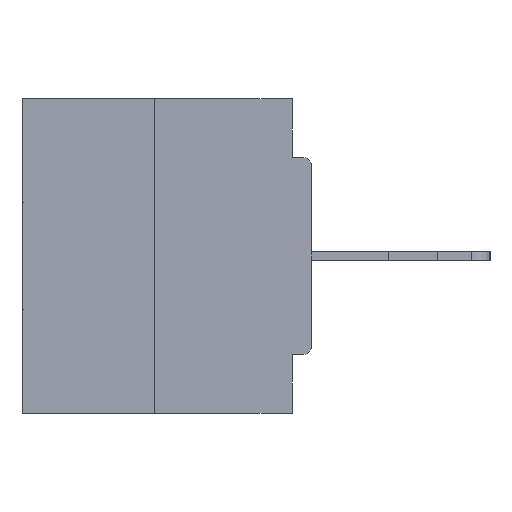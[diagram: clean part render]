
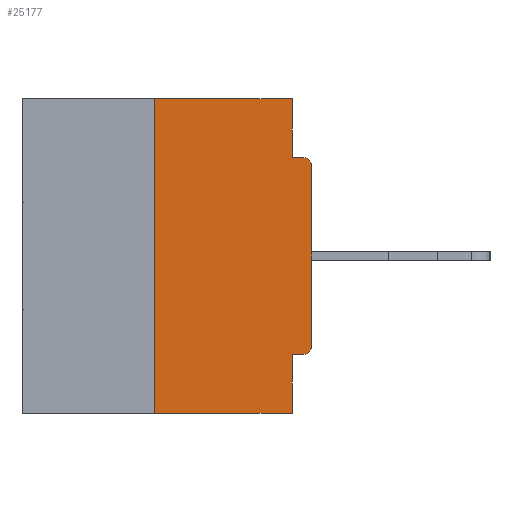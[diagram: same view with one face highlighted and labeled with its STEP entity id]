
A CAD part, left-side view. The second image highlights one B-rep face of the part: STEP entity #25177.
In plain terms, the highlighted planar face has unit normal (-1, 0, 0).
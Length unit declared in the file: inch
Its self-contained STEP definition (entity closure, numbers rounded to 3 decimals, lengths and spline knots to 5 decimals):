
#40 = EDGE_CURVE ( 'NONE', #13439, #9041, #28304, .T. ) ;
#53 = CARTESIAN_POINT ( 'NONE',  ( 0., 0.031, 0. ) ) ;
#135 = ORIENTED_EDGE ( 'NONE', *, *, #31117, .F. ) ;
#334 = CARTESIAN_POINT ( 'NONE',  ( 0., 0.031, 0. ) ) ;
#737 = EDGE_CURVE ( 'NONE', #1061, #24959, #9165, .T. ) ;
#854 = EDGE_CURVE ( 'NONE', #18904, #9041, #8655, .T. ) ;
#1061 = VERTEX_POINT ( 'NONE', #24349 ) ;
#1246 = DIRECTION ( 'NONE',  ( 0., 0., -1. ) ) ;
#1513 = VECTOR ( 'NONE', #6219, 39.37008 ) ;
#1588 = VECTOR ( 'NONE', #11652, 39.37008 ) ;
#2997 = EDGE_LOOP ( 'NONE', ( #18141, #19360, #4685, #22809, #18071, #13295, #12300, #4319, #24448, #135 ) ) ;
#3257 = DIRECTION ( 'NONE',  ( 0., 0., 1. ) ) ;
#4319 = ORIENTED_EDGE ( 'NONE', *, *, #25153, .T. ) ;
#4685 = ORIENTED_EDGE ( 'NONE', *, *, #854, .T. ) ;
#5318 = DIRECTION ( 'NONE',  ( 0., 0., -1. ) ) ;
#5528 = LINE ( 'NONE', #16501, #17212 ) ;
#6044 = CARTESIAN_POINT ( 'NONE',  ( 0., 0.46, -0.5 ) ) ;
#6219 = DIRECTION ( 'NONE',  ( 0., -1., 0. ) ) ;
#7610 = CARTESIAN_POINT ( 'NONE',  ( 0., 0., -0.4065 ) ) ;
#8655 = LINE ( 'NONE', #6044, #16555 ) ;
#9040 = VECTOR ( 'NONE', #1246, 39.37008 ) ;
#9041 = VERTEX_POINT ( 'NONE', #32996 ) ;
#9165 = LINE ( 'NONE', #25255, #1513 ) ;
#9219 = CARTESIAN_POINT ( 'NONE',  ( 0., 0., 0. ) ) ;
#9631 = CARTESIAN_POINT ( 'NONE',  ( 0., 0.25, -0.5 ) ) ;
#9983 = EDGE_CURVE ( 'NONE', #22414, #21853, #27924, .T. ) ;
#10182 = VECTOR ( 'NONE', #23954, 39.37008 ) ;
#10541 = CARTESIAN_POINT ( 'NONE',  ( 0., 0.015, -0.3915 ) ) ;
#11055 = VERTEX_POINT ( 'NONE', #11206 ) ;
#11206 = CARTESIAN_POINT ( 'NONE',  ( 0., 0.25, 0. ) ) ;
#11652 = DIRECTION ( 'NONE',  ( 0., 0., -1. ) ) ;
#11832 = DIRECTION ( 'NONE',  ( 0., 0., 1. ) ) ;
#12300 = ORIENTED_EDGE ( 'NONE', *, *, #9983, .T. ) ;
#13295 = ORIENTED_EDGE ( 'NONE', *, *, #13466, .T. ) ;
#13439 = VERTEX_POINT ( 'NONE', #15628 ) ;
#13466 = EDGE_CURVE ( 'NONE', #27316, #22414, #32610, .T. ) ;
#13702 = DIRECTION ( 'NONE',  ( 0., 1., 0. ) ) ;
#14449 = LINE ( 'NONE', #53, #1588 ) ;
#15037 = CARTESIAN_POINT ( 'NONE',  ( 0., 0., -0.3915 ) ) ;
#15628 = CARTESIAN_POINT ( 'NONE',  ( 0., 0.031, -0.4065 ) ) ;
#16501 = CARTESIAN_POINT ( 'NONE',  ( 0., 0.25, 0. ) ) ;
#16555 = VECTOR ( 'NONE', #29968, 39.37008 ) ;
#16938 = CARTESIAN_POINT ( 'NONE',  ( 0., 0.015, -0.1085 ) ) ;
#17109 = DIRECTION ( 'NONE',  ( 1., 0., 0. ) ) ;
#17212 = VECTOR ( 'NONE', #3257, 39.37008 ) ;
#18071 = ORIENTED_EDGE ( 'NONE', *, *, #22909, .F. ) ;
#18141 = ORIENTED_EDGE ( 'NONE', *, *, #24982, .F. ) ;
#18779 = EDGE_CURVE ( 'NONE', #18904, #11055, #5528, .T. ) ;
#18810 = VECTOR ( 'NONE', #11832, 39.37008 ) ;
#18904 = VERTEX_POINT ( 'NONE', #9631 ) ;
#19360 = ORIENTED_EDGE ( 'NONE', *, *, #18779, .F. ) ;
#19716 = DIRECTION ( 'NONE',  ( 0., 0., -1. ) ) ;
#21312 = VECTOR ( 'NONE', #13702, 39.37008 ) ;
#21853 = VERTEX_POINT ( 'NONE', #27475 ) ;
#22016 = AXIS2_PLACEMENT_3D ( 'NONE', #10541, #24009, #5318 ) ;
#22414 = VERTEX_POINT ( 'NONE', #15037 ) ;
#22809 = ORIENTED_EDGE ( 'NONE', *, *, #40, .F. ) ;
#22909 = EDGE_CURVE ( 'NONE', #27316, #13439, #32033, .T. ) ;
#23954 = DIRECTION ( 'NONE',  ( 0., -1., 0. ) ) ;
#24009 = DIRECTION ( 'NONE',  ( -1., 0., 0. ) ) ;
#24349 = CARTESIAN_POINT ( 'NONE',  ( 0., 0.031, -0.0935 ) ) ;
#24448 = ORIENTED_EDGE ( 'NONE', *, *, #737, .F. ) ;
#24477 = FACE_OUTER_BOUND ( 'NONE', #2997, .T. ) ;
#24959 = VERTEX_POINT ( 'NONE', #26750 ) ;
#24982 = EDGE_CURVE ( 'NONE', #11055, #33859, #26402, .T. ) ;
#24991 = PLANE ( 'NONE',  #34207 ) ;
#25153 = EDGE_CURVE ( 'NONE', #21853, #24959, #30843, .T. ) ;
#25177 = ADVANCED_FACE ( 'NONE', ( #24477 ), #24991, .F. ) ;
#25255 = CARTESIAN_POINT ( 'NONE',  ( 0., 0., -0.0935 ) ) ;
#25531 = CARTESIAN_POINT ( 'NONE',  ( 0., 0.015, -0.4065 ) ) ;
#26402 = LINE ( 'NONE', #29192, #10182 ) ;
#26750 = CARTESIAN_POINT ( 'NONE',  ( 0., 0.015, -0.0935 ) ) ;
#27316 = VERTEX_POINT ( 'NONE', #25531 ) ;
#27475 = CARTESIAN_POINT ( 'NONE',  ( 0., 0., -0.1085 ) ) ;
#27591 = DIRECTION ( 'NONE',  ( -1., 0., 0. ) ) ;
#27924 = LINE ( 'NONE', #9219, #18810 ) ;
#28071 = AXIS2_PLACEMENT_3D ( 'NONE', #16938, #27591, #19716 ) ;
#28289 = CARTESIAN_POINT ( 'NONE',  ( 0., 0.46, 0. ) ) ;
#28304 = LINE ( 'NONE', #30570, #9040 ) ;
#29192 = CARTESIAN_POINT ( 'NONE',  ( 0., 0.46, 0. ) ) ;
#29968 = DIRECTION ( 'NONE',  ( 0., -1., 0. ) ) ;
#30570 = CARTESIAN_POINT ( 'NONE',  ( 0., 0.031, -0.5 ) ) ;
#30843 = CIRCLE ( 'NONE', #28071, 0.015 ) ;
#30887 = DIRECTION ( 'NONE',  ( 0., 0., -1. ) ) ;
#31117 = EDGE_CURVE ( 'NONE', #33859, #1061, #14449, .T. ) ;
#32033 = LINE ( 'NONE', #7610, #21312 ) ;
#32610 = CIRCLE ( 'NONE', #22016, 0.015 ) ;
#32996 = CARTESIAN_POINT ( 'NONE',  ( 0., 0.031, -0.5 ) ) ;
#33859 = VERTEX_POINT ( 'NONE', #334 ) ;
#34207 = AXIS2_PLACEMENT_3D ( 'NONE', #28289, #17109, #30887 ) ;
